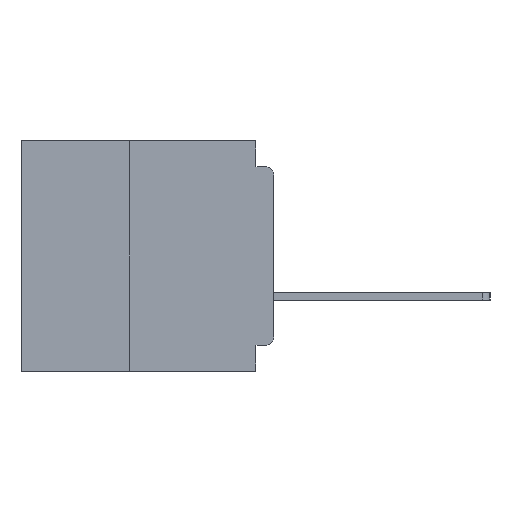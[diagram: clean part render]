
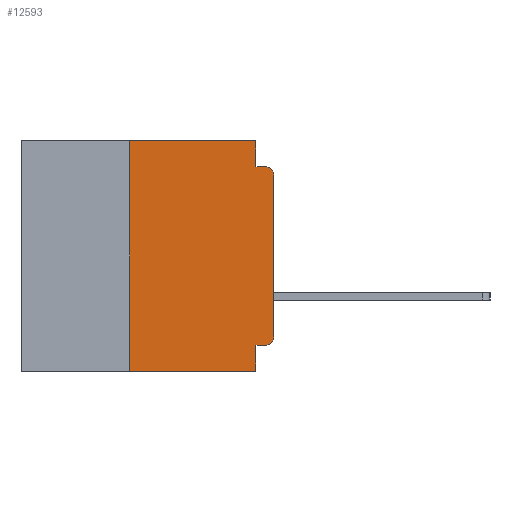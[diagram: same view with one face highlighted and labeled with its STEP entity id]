
A CAD part, left-side view. The second image highlights one B-rep face of the part: STEP entity #12593.
In plain terms, the highlighted planar face has unit normal (-1, 0, 0).
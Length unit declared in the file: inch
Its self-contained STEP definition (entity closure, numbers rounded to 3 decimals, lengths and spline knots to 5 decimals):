
#452 = ORIENTED_EDGE ( 'NONE', *, *, #6549, .F. ) ;
#691 = EDGE_CURVE ( 'NONE', #10210, #26636, #22953, .T. ) ;
#1492 = CARTESIAN_POINT ( 'NONE',  ( 0., 0.437, 0. ) ) ;
#2782 = VECTOR ( 'NONE', #35533, 39.37008 ) ;
#3183 = EDGE_CURVE ( 'NONE', #6914, #9775, #14823, .T. ) ;
#4417 = EDGE_CURVE ( 'NONE', #11059, #21653, #17433, .T. ) ;
#4477 = CARTESIAN_POINT ( 'NONE',  ( 0., 0.437, -0.4 ) ) ;
#5872 = VECTOR ( 'NONE', #13893, 39.37008 ) ;
#6138 = ORIENTED_EDGE ( 'NONE', *, *, #27820, .T. ) ;
#6335 = ORIENTED_EDGE ( 'NONE', *, *, #15038, .F. ) ;
#6549 = EDGE_CURVE ( 'NONE', #33550, #29559, #24911, .T. ) ;
#6652 = VECTOR ( 'NONE', #11517, 39.37008 ) ;
#6914 = VERTEX_POINT ( 'NONE', #12862 ) ;
#6983 = CARTESIAN_POINT ( 'NONE',  ( 0., 0.015, -0.34 ) ) ;
#8254 = AXIS2_PLACEMENT_3D ( 'NONE', #6983, #27132, #9899 ) ;
#8522 = ORIENTED_EDGE ( 'NONE', *, *, #18021, .T. ) ;
#8841 = VECTOR ( 'NONE', #18935, 39.37008 ) ;
#9304 = DIRECTION ( 'NONE',  ( -1., 0., 0. ) ) ;
#9458 = CARTESIAN_POINT ( 'NONE',  ( 0., 0.031, -0.4 ) ) ;
#9775 = VERTEX_POINT ( 'NONE', #33901 ) ;
#9899 = DIRECTION ( 'NONE',  ( 0., 0., -1. ) ) ;
#10210 = VERTEX_POINT ( 'NONE', #10612 ) ;
#10272 = EDGE_CURVE ( 'NONE', #26636, #33550, #34731, .T. ) ;
#10355 = VERTEX_POINT ( 'NONE', #22970 ) ;
#10612 = CARTESIAN_POINT ( 'NONE',  ( 0., 0.25, 0. ) ) ;
#11059 = VERTEX_POINT ( 'NONE', #31814 ) ;
#11451 = LINE ( 'NONE', #24008, #2782 ) ;
#11517 = DIRECTION ( 'NONE',  ( 0., -1., 0. ) ) ;
#12542 = CIRCLE ( 'NONE', #34661, 0.015 ) ;
#12593 = ADVANCED_FACE ( 'NONE', ( #23325 ), #23310, .F. ) ;
#12744 = AXIS2_PLACEMENT_3D ( 'NONE', #34721, #31962, #14745 ) ;
#12862 = CARTESIAN_POINT ( 'NONE',  ( 0., 0.015, -0.355 ) ) ;
#13353 = CARTESIAN_POINT ( 'NONE',  ( 0., 0.031, -0.4 ) ) ;
#13893 = DIRECTION ( 'NONE',  ( 0., 0., -1. ) ) ;
#14377 = ORIENTED_EDGE ( 'NONE', *, *, #4417, .T. ) ;
#14745 = DIRECTION ( 'NONE',  ( 0., 0., -1. ) ) ;
#14823 = LINE ( 'NONE', #22980, #29220 ) ;
#15038 = EDGE_CURVE ( 'NONE', #11059, #10210, #31943, .T. ) ;
#16654 = VECTOR ( 'NONE', #36188, 39.37008 ) ;
#17433 = LINE ( 'NONE', #4477, #8841 ) ;
#17793 = ORIENTED_EDGE ( 'NONE', *, *, #3183, .F. ) ;
#18021 = EDGE_CURVE ( 'NONE', #27214, #10355, #11451, .T. ) ;
#18306 = LINE ( 'NONE', #9458, #32667 ) ;
#18702 = CARTESIAN_POINT ( 'NONE',  ( 0., 0.031, 0. ) ) ;
#18935 = DIRECTION ( 'NONE',  ( 0., -1., 0. ) ) ;
#19022 = CARTESIAN_POINT ( 'NONE',  ( 0., 0.25, -0.4 ) ) ;
#21653 = VERTEX_POINT ( 'NONE', #13353 ) ;
#22953 = LINE ( 'NONE', #1492, #6652 ) ;
#22970 = CARTESIAN_POINT ( 'NONE',  ( 0., 0., -0.06 ) ) ;
#22980 = CARTESIAN_POINT ( 'NONE',  ( 0., 0., -0.355 ) ) ;
#23230 = CARTESIAN_POINT ( 'NONE',  ( 0., 0.015, -0.045 ) ) ;
#23260 = DIRECTION ( 'NONE',  ( 0., 1., 0. ) ) ;
#23310 = PLANE ( 'NONE',  #12744 ) ;
#23325 = FACE_OUTER_BOUND ( 'NONE', #32802, .T. ) ;
#23920 = ORIENTED_EDGE ( 'NONE', *, *, #35294, .T. ) ;
#23968 = DIRECTION ( 'NONE',  ( 0., 0., -1. ) ) ;
#24008 = CARTESIAN_POINT ( 'NONE',  ( 0., 0., 0. ) ) ;
#24821 = CARTESIAN_POINT ( 'NONE',  ( 0., 0.031, -0.045 ) ) ;
#24911 = LINE ( 'NONE', #34267, #25808 ) ;
#25626 = DIRECTION ( 'NONE',  ( 0., -1., 0. ) ) ;
#25808 = VECTOR ( 'NONE', #25626, 39.37008 ) ;
#25969 = ORIENTED_EDGE ( 'NONE', *, *, #36525, .F. ) ;
#26569 = CARTESIAN_POINT ( 'NONE',  ( 0., 0.015, -0.06 ) ) ;
#26636 = VERTEX_POINT ( 'NONE', #18702 ) ;
#27132 = DIRECTION ( 'NONE',  ( -1., 0., 0. ) ) ;
#27214 = VERTEX_POINT ( 'NONE', #32709 ) ;
#27820 = EDGE_CURVE ( 'NONE', #6914, #27214, #33726, .T. ) ;
#28654 = ORIENTED_EDGE ( 'NONE', *, *, #10272, .F. ) ;
#29220 = VECTOR ( 'NONE', #23260, 39.37008 ) ;
#29452 = DIRECTION ( 'NONE',  ( 0., 0., -1. ) ) ;
#29559 = VERTEX_POINT ( 'NONE', #23230 ) ;
#31134 = CARTESIAN_POINT ( 'NONE',  ( 0., 0.031, 0. ) ) ;
#31814 = CARTESIAN_POINT ( 'NONE',  ( 0., 0.25, -0.4 ) ) ;
#31943 = LINE ( 'NONE', #19022, #16654 ) ;
#31962 = DIRECTION ( 'NONE',  ( 1., 0., 0. ) ) ;
#32667 = VECTOR ( 'NONE', #23968, 39.37008 ) ;
#32709 = CARTESIAN_POINT ( 'NONE',  ( 0., 0., -0.34 ) ) ;
#32802 = EDGE_LOOP ( 'NONE', ( #8522, #23920, #452, #28654, #33531, #6335, #14377, #25969, #17793, #6138 ) ) ;
#33531 = ORIENTED_EDGE ( 'NONE', *, *, #691, .F. ) ;
#33550 = VERTEX_POINT ( 'NONE', #24821 ) ;
#33726 = CIRCLE ( 'NONE', #8254, 0.015 ) ;
#33901 = CARTESIAN_POINT ( 'NONE',  ( 0., 0.031, -0.355 ) ) ;
#34267 = CARTESIAN_POINT ( 'NONE',  ( 0., 0., -0.045 ) ) ;
#34661 = AXIS2_PLACEMENT_3D ( 'NONE', #26569, #9304, #29452 ) ;
#34721 = CARTESIAN_POINT ( 'NONE',  ( 0., 0.437, 0. ) ) ;
#34731 = LINE ( 'NONE', #31134, #5872 ) ;
#35294 = EDGE_CURVE ( 'NONE', #10355, #29559, #12542, .T. ) ;
#35533 = DIRECTION ( 'NONE',  ( 0., 0., 1. ) ) ;
#36188 = DIRECTION ( 'NONE',  ( 0., 0., 1. ) ) ;
#36525 = EDGE_CURVE ( 'NONE', #9775, #21653, #18306, .T. ) ;
